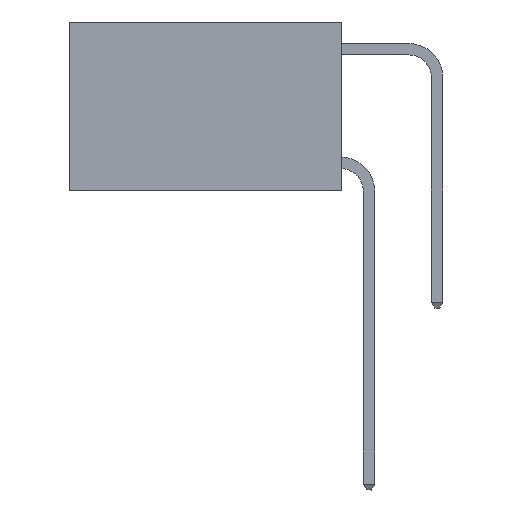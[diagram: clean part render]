
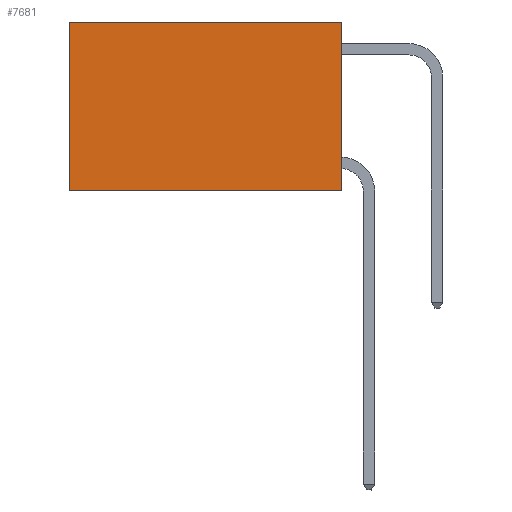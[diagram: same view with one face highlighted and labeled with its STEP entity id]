
A CAD part, left-side view. The second image highlights one B-rep face of the part: STEP entity #7681.
In plain terms, the highlighted planar face has unit normal (-1, 0, 0).
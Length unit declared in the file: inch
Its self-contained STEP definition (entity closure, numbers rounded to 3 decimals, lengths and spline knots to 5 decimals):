
#209 = VERTEX_POINT ( 'NONE', #18123 ) ;
#978 = CARTESIAN_POINT ( 'NONE',  ( 0.2625, 0., 0. ) ) ;
#2425 = LINE ( 'NONE', #2787, #11683 ) ;
#2787 = CARTESIAN_POINT ( 'NONE',  ( 0.2625, 0., -0.37 ) ) ;
#2909 = DIRECTION ( 'NONE',  ( 1., 0., 0. ) ) ;
#3426 = VECTOR ( 'NONE', #3527, 39.37008 ) ;
#3527 = DIRECTION ( 'NONE',  ( 0., 0., -1. ) ) ;
#3538 = EDGE_CURVE ( 'NONE', #9795, #209, #22437, .T. ) ;
#4754 = ORIENTED_EDGE ( 'NONE', *, *, #15065, .T. ) ;
#7280 = CARTESIAN_POINT ( 'NONE',  ( 0.2625, 0., -0.37 ) ) ;
#7328 = VECTOR ( 'NONE', #8033, 39.37008 ) ;
#7613 = CARTESIAN_POINT ( 'NONE',  ( 0.2625, 0.6, 0. ) ) ;
#7681 = ADVANCED_FACE ( 'NONE', ( #14501 ), #20003, .F. ) ;
#8033 = DIRECTION ( 'NONE',  ( 0., 0., -1. ) ) ;
#8279 = DIRECTION ( 'NONE',  ( 0., 1., 0. ) ) ;
#9208 = ORIENTED_EDGE ( 'NONE', *, *, #3538, .T. ) ;
#9263 = VECTOR ( 'NONE', #8279, 39.37008 ) ;
#9795 = VERTEX_POINT ( 'NONE', #7613 ) ;
#9919 = DIRECTION ( 'NONE',  ( 0., 1., 0. ) ) ;
#11683 = VECTOR ( 'NONE', #9919, 39.37008 ) ;
#11931 = VERTEX_POINT ( 'NONE', #7280 ) ;
#12030 = CARTESIAN_POINT ( 'NONE',  ( 0.2625, 0., 0. ) ) ;
#12401 = DIRECTION ( 'NONE',  ( 0., 0., -1. ) ) ;
#12581 = CARTESIAN_POINT ( 'NONE',  ( 0.2625, 0., 0. ) ) ;
#13697 = EDGE_CURVE ( 'NONE', #13968, #11931, #19566, .T. ) ;
#13968 = VERTEX_POINT ( 'NONE', #12030 ) ;
#14465 = EDGE_CURVE ( 'NONE', #11931, #209, #2425, .T. ) ;
#14501 = FACE_OUTER_BOUND ( 'NONE', #19337, .T. ) ;
#15065 = EDGE_CURVE ( 'NONE', #13968, #9795, #19697, .T. ) ;
#17601 = ORIENTED_EDGE ( 'NONE', *, *, #14465, .F. ) ;
#18123 = CARTESIAN_POINT ( 'NONE',  ( 0.2625, 0.6, -0.37 ) ) ;
#19337 = EDGE_LOOP ( 'NONE', ( #9208, #17601, #20330, #4754 ) ) ;
#19566 = LINE ( 'NONE', #978, #7328 ) ;
#19697 = LINE ( 'NONE', #12581, #9263 ) ;
#20003 = PLANE ( 'NONE',  #22161 ) ;
#20330 = ORIENTED_EDGE ( 'NONE', *, *, #13697, .F. ) ;
#20354 = CARTESIAN_POINT ( 'NONE',  ( 0.2625, 0.6, 0. ) ) ;
#21955 = CARTESIAN_POINT ( 'NONE',  ( 0.2625, 0., 0. ) ) ;
#22161 = AXIS2_PLACEMENT_3D ( 'NONE', #21955, #2909, #12401 ) ;
#22437 = LINE ( 'NONE', #20354, #3426 ) ;
